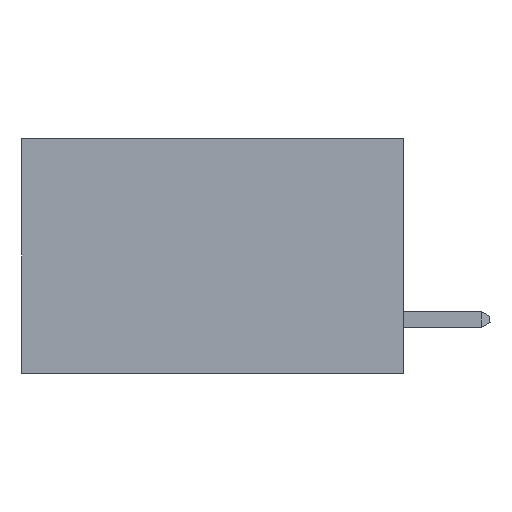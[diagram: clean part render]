
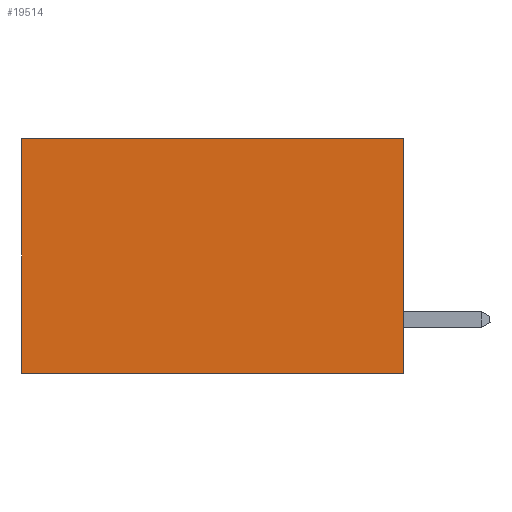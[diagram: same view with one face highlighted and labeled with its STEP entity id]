
A CAD part, left-side view. The second image highlights one B-rep face of the part: STEP entity #19514.
In plain terms, the highlighted planar face has unit normal (-1, 0, 0).
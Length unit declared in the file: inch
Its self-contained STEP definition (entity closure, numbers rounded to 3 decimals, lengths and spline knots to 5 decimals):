
#395 = DIRECTION ( 'NONE',  ( 0., 0., -1. ) ) ;
#2425 = EDGE_CURVE ( 'NONE', #35624, #18779, #34704, .T. ) ;
#3067 = LINE ( 'NONE', #11672, #11575 ) ;
#3734 = FACE_OUTER_BOUND ( 'NONE', #20090, .T. ) ;
#4097 = EDGE_CURVE ( 'NONE', #13072, #33012, #15564, .T. ) ;
#7013 = VECTOR ( 'NONE', #395, 39.37008 ) ;
#7218 = VECTOR ( 'NONE', #26076, 39.37008 ) ;
#7674 = DIRECTION ( 'NONE',  ( 0., 1., 0. ) ) ;
#10257 = CARTESIAN_POINT ( 'NONE',  ( 0.2875, 0.6, 0. ) ) ;
#10445 = CARTESIAN_POINT ( 'NONE',  ( 0.2875, 0.6, -0.37 ) ) ;
#11575 = VECTOR ( 'NONE', #7674, 39.37008 ) ;
#11672 = CARTESIAN_POINT ( 'NONE',  ( 0.2875, 0., 0. ) ) ;
#11955 = DIRECTION ( 'NONE',  ( 0., 0., -1. ) ) ;
#12950 = EDGE_CURVE ( 'NONE', #18779, #33012, #25537, .T. ) ;
#13072 = VERTEX_POINT ( 'NONE', #10257 ) ;
#13356 = CARTESIAN_POINT ( 'NONE',  ( 0.2875, 0., -0.37 ) ) ;
#13862 = CARTESIAN_POINT ( 'NONE',  ( 0.2875, 0., 0. ) ) ;
#15564 = LINE ( 'NONE', #22293, #7013 ) ;
#16940 = DIRECTION ( 'NONE',  ( 1., 0., 0. ) ) ;
#17560 = ORIENTED_EDGE ( 'NONE', *, *, #12950, .F. ) ;
#18779 = VERTEX_POINT ( 'NONE', #36124 ) ;
#19514 = ADVANCED_FACE ( 'NONE', ( #3734 ), #35504, .F. ) ;
#20090 = EDGE_LOOP ( 'NONE', ( #44316, #17560, #32001, #33244 ) ) ;
#22293 = CARTESIAN_POINT ( 'NONE',  ( 0.2875, 0.6, 0. ) ) ;
#25537 = LINE ( 'NONE', #13356, #38735 ) ;
#26076 = DIRECTION ( 'NONE',  ( 0., 0., -1. ) ) ;
#32001 = ORIENTED_EDGE ( 'NONE', *, *, #2425, .F. ) ;
#33012 = VERTEX_POINT ( 'NONE', #10445 ) ;
#33244 = ORIENTED_EDGE ( 'NONE', *, *, #45793, .T. ) ;
#34704 = LINE ( 'NONE', #44572, #7218 ) ;
#34991 = DIRECTION ( 'NONE',  ( 0., 1., 0. ) ) ;
#35504 = PLANE ( 'NONE',  #37553 ) ;
#35624 = VERTEX_POINT ( 'NONE', #42508 ) ;
#36124 = CARTESIAN_POINT ( 'NONE',  ( 0.2875, 0., -0.37 ) ) ;
#37553 = AXIS2_PLACEMENT_3D ( 'NONE', #13862, #16940, #11955 ) ;
#38735 = VECTOR ( 'NONE', #34991, 39.37008 ) ;
#42508 = CARTESIAN_POINT ( 'NONE',  ( 0.2875, 0., 0. ) ) ;
#44316 = ORIENTED_EDGE ( 'NONE', *, *, #4097, .T. ) ;
#44572 = CARTESIAN_POINT ( 'NONE',  ( 0.2875, 0., 0. ) ) ;
#45793 = EDGE_CURVE ( 'NONE', #35624, #13072, #3067, .T. ) ;
